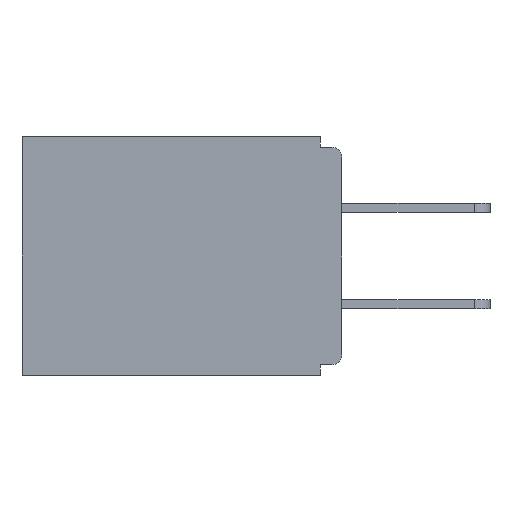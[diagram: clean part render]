
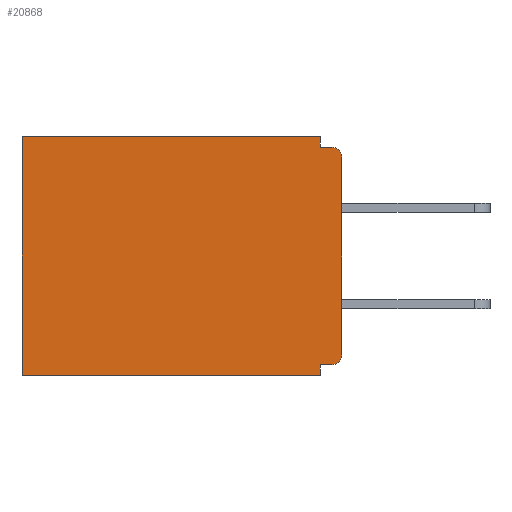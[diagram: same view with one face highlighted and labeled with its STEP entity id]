
A CAD part, left-side view. The second image highlights one B-rep face of the part: STEP entity #20868.
In plain terms, the highlighted planar face has unit normal (-1, 0, 0).
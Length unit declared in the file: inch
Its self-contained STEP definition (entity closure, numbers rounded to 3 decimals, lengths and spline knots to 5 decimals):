
#102 = EDGE_CURVE ( 'NONE', #19788, #10099, #6288, .T. ) ;
#279 = DIRECTION ( 'NONE',  ( 0., 0., -1. ) ) ;
#743 = CARTESIAN_POINT ( 'NONE',  ( 0.298, 0.031, -0.328 ) ) ;
#917 = ORIENTED_EDGE ( 'NONE', *, *, #4127, .T. ) ;
#1670 = ORIENTED_EDGE ( 'NONE', *, *, #2860, .F. ) ;
#1795 = CARTESIAN_POINT ( 'NONE',  ( 0.298, 0., 0. ) ) ;
#2374 = EDGE_CURVE ( 'NONE', #2890, #19249, #26034, .T. ) ;
#2860 = EDGE_CURVE ( 'NONE', #2890, #19788, #19042, .T. ) ;
#2890 = VERTEX_POINT ( 'NONE', #14279 ) ;
#3876 = CARTESIAN_POINT ( 'NONE',  ( 0.298, 0., 0. ) ) ;
#3889 = LINE ( 'NONE', #23610, #19133 ) ;
#4127 = EDGE_CURVE ( 'NONE', #6356, #11900, #19600, .T. ) ;
#4416 = CARTESIAN_POINT ( 'NONE',  ( 0.298, 0., -0.343 ) ) ;
#5209 = ORIENTED_EDGE ( 'NONE', *, *, #11208, .T. ) ;
#5546 = CARTESIAN_POINT ( 'NONE',  ( 0.298, 0.46, -0.343 ) ) ;
#5931 = DIRECTION ( 'NONE',  ( 0., 0., -1. ) ) ;
#6084 = CARTESIAN_POINT ( 'NONE',  ( 0.298, 0.46, 0. ) ) ;
#6096 = EDGE_CURVE ( 'NONE', #27028, #6561, #3889, .T. ) ;
#6288 = LINE ( 'NONE', #21592, #9739 ) ;
#6356 = VERTEX_POINT ( 'NONE', #6084 ) ;
#6378 = VECTOR ( 'NONE', #28661, 39.37008 ) ;
#6500 = ORIENTED_EDGE ( 'NONE', *, *, #102, .F. ) ;
#6561 = VERTEX_POINT ( 'NONE', #11267 ) ;
#6850 = VECTOR ( 'NONE', #19910, 39.37008 ) ;
#7441 = VERTEX_POINT ( 'NONE', #9667 ) ;
#8824 = EDGE_CURVE ( 'NONE', #10099, #11900, #26268, .T. ) ;
#9667 = CARTESIAN_POINT ( 'NONE',  ( 0.298, 0.031, 0. ) ) ;
#9739 = VECTOR ( 'NONE', #25951, 39.37008 ) ;
#10099 = VERTEX_POINT ( 'NONE', #15254 ) ;
#10566 = DIRECTION ( 'NONE',  ( 0., -1., 0. ) ) ;
#10651 = CARTESIAN_POINT ( 'NONE',  ( 0.298, 0., -0.03 ) ) ;
#10874 = EDGE_LOOP ( 'NONE', ( #5209, #24366, #14699, #18597, #917, #23981, #6500, #1670, #25373, #20015 ) ) ;
#11208 = EDGE_CURVE ( 'NONE', #21717, #6561, #13381, .T. ) ;
#11267 = CARTESIAN_POINT ( 'NONE',  ( 0.298, 0.015, -0.015 ) ) ;
#11900 = VERTEX_POINT ( 'NONE', #5546 ) ;
#11929 = DIRECTION ( 'NONE',  ( -1., 0., 0. ) ) ;
#11939 = DIRECTION ( 'NONE',  ( 0., 1., 0. ) ) ;
#13054 = LINE ( 'NONE', #1795, #6850 ) ;
#13381 = CIRCLE ( 'NONE', #21087, 0.015 ) ;
#14170 = DIRECTION ( 'NONE',  ( 0., 0., -1. ) ) ;
#14279 = CARTESIAN_POINT ( 'NONE',  ( 0.298, 0.015, -0.328 ) ) ;
#14489 = VECTOR ( 'NONE', #16626, 39.37008 ) ;
#14699 = ORIENTED_EDGE ( 'NONE', *, *, #17997, .F. ) ;
#14964 = DIRECTION ( 'NONE',  ( 0., 0., -1. ) ) ;
#14970 = DIRECTION ( 'NONE',  ( 0., 0., -1. ) ) ;
#15114 = CARTESIAN_POINT ( 'NONE',  ( 0.298, 0.031, -0.343 ) ) ;
#15166 = PLANE ( 'NONE',  #16137 ) ;
#15254 = CARTESIAN_POINT ( 'NONE',  ( 0.298, 0.031, -0.343 ) ) ;
#15948 = EDGE_CURVE ( 'NONE', #7441, #6356, #13054, .T. ) ;
#16137 = AXIS2_PLACEMENT_3D ( 'NONE', #3876, #23762, #14964 ) ;
#16626 = DIRECTION ( 'NONE',  ( 0., 1., 0. ) ) ;
#16648 = FACE_OUTER_BOUND ( 'NONE', #10874, .T. ) ;
#16742 = EDGE_CURVE ( 'NONE', #21717, #19249, #24882, .T. ) ;
#17145 = DIRECTION ( 'NONE',  ( -1., 0., 0. ) ) ;
#17853 = VECTOR ( 'NONE', #5931, 39.37008 ) ;
#17997 = EDGE_CURVE ( 'NONE', #7441, #27028, #23769, .T. ) ;
#18597 = ORIENTED_EDGE ( 'NONE', *, *, #15948, .T. ) ;
#18961 = AXIS2_PLACEMENT_3D ( 'NONE', #24060, #17145, #14970 ) ;
#19042 = LINE ( 'NONE', #27630, #14489 ) ;
#19133 = VECTOR ( 'NONE', #10566, 39.37008 ) ;
#19249 = VERTEX_POINT ( 'NONE', #21340 ) ;
#19423 = CARTESIAN_POINT ( 'NONE',  ( 0.298, 0.031, -0.015 ) ) ;
#19600 = LINE ( 'NONE', #24125, #6378 ) ;
#19788 = VERTEX_POINT ( 'NONE', #743 ) ;
#19910 = DIRECTION ( 'NONE',  ( 0., 1., 0. ) ) ;
#20015 = ORIENTED_EDGE ( 'NONE', *, *, #16742, .F. ) ;
#20868 = ADVANCED_FACE ( 'NONE', ( #16648 ), #15166, .F. ) ;
#21087 = AXIS2_PLACEMENT_3D ( 'NONE', #23059, #11929, #14170 ) ;
#21340 = CARTESIAN_POINT ( 'NONE',  ( 0.298, 0., -0.313 ) ) ;
#21592 = CARTESIAN_POINT ( 'NONE',  ( 0.298, 0.031, -0.343 ) ) ;
#21717 = VERTEX_POINT ( 'NONE', #10651 ) ;
#21761 = VECTOR ( 'NONE', #11939, 39.37008 ) ;
#23059 = CARTESIAN_POINT ( 'NONE',  ( 0.298, 0.015, -0.03 ) ) ;
#23610 = CARTESIAN_POINT ( 'NONE',  ( 0.298, 0., -0.015 ) ) ;
#23762 = DIRECTION ( 'NONE',  ( 1., 0., 0. ) ) ;
#23769 = LINE ( 'NONE', #15114, #17853 ) ;
#23981 = ORIENTED_EDGE ( 'NONE', *, *, #8824, .F. ) ;
#24060 = CARTESIAN_POINT ( 'NONE',  ( 0.298, 0.015, -0.313 ) ) ;
#24125 = CARTESIAN_POINT ( 'NONE',  ( 0.298, 0.46, 0. ) ) ;
#24366 = ORIENTED_EDGE ( 'NONE', *, *, #6096, .F. ) ;
#24882 = LINE ( 'NONE', #26860, #28357 ) ;
#25373 = ORIENTED_EDGE ( 'NONE', *, *, #2374, .T. ) ;
#25951 = DIRECTION ( 'NONE',  ( 0., 0., -1. ) ) ;
#26034 = CIRCLE ( 'NONE', #18961, 0.015 ) ;
#26268 = LINE ( 'NONE', #4416, #21761 ) ;
#26860 = CARTESIAN_POINT ( 'NONE',  ( 0.298, 0., 0. ) ) ;
#27028 = VERTEX_POINT ( 'NONE', #19423 ) ;
#27630 = CARTESIAN_POINT ( 'NONE',  ( 0.298, 0., -0.328 ) ) ;
#28357 = VECTOR ( 'NONE', #279, 39.37008 ) ;
#28661 = DIRECTION ( 'NONE',  ( 0., 0., -1. ) ) ;
